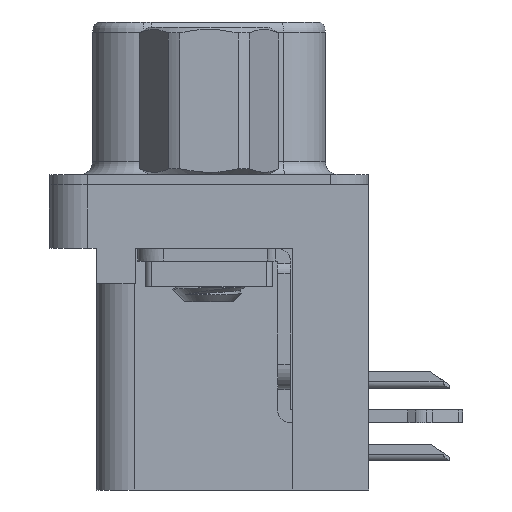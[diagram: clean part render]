
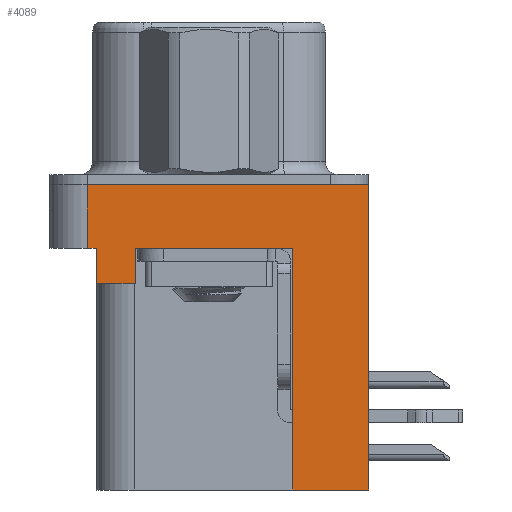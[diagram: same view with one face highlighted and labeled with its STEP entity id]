
A CAD part, left-side view. The second image highlights one B-rep face of the part: STEP entity #4089.
In plain terms, the highlighted planar face has unit normal (-1, 0, 0).
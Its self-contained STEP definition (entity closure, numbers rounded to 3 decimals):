
#299 = VECTOR ( 'NONE', #5499, 1000. ) ;
#328 = CARTESIAN_POINT ( 'NONE',  ( -2.935, -3.295, -12. ) ) ;
#560 = LINE ( 'NONE', #13703, #13429 ) ;
#997 = EDGE_CURVE ( 'NONE', #20167, #11208, #11952, .T. ) ;
#1249 = EDGE_CURVE ( 'NONE', #15625, #7028, #13150, .T. ) ;
#1356 = CARTESIAN_POINT ( 'NONE',  ( -2.935, 2.895, -2.5 ) ) ;
#1604 = CARTESIAN_POINT ( 'NONE',  ( -2.935, 2.895, -3.9 ) ) ;
#2336 = FACE_OUTER_BOUND ( 'NONE', #5915, .T. ) ;
#2530 = LINE ( 'NONE', #23417, #11788 ) ;
#2754 = ORIENTED_EDGE ( 'NONE', *, *, #14510, .F. ) ;
#2877 = VERTEX_POINT ( 'NONE', #21437 ) ;
#2952 = CARTESIAN_POINT ( 'NONE',  ( -2.935, -6.275, -2.5 ) ) ;
#3933 = ORIENTED_EDGE ( 'NONE', *, *, #22771, .F. ) ;
#4046 = EDGE_CURVE ( 'NONE', #7547, #11208, #22954, .T. ) ;
#4089 = ADVANCED_FACE ( 'NONE', ( #2336 ), #18401, .T. ) ;
#4191 = CARTESIAN_POINT ( 'NONE',  ( -2.935, -3.295, -2.5 ) ) ;
#4959 = CARTESIAN_POINT ( 'NONE',  ( -2.935, -6.275, -2.5 ) ) ;
#5136 = ORIENTED_EDGE ( 'NONE', *, *, #6308, .F. ) ;
#5379 = CARTESIAN_POINT ( 'NONE',  ( -2.935, 4.775, -2.5 ) ) ;
#5499 = DIRECTION ( 'NONE',  ( 0., 0., 1. ) ) ;
#5915 = EDGE_LOOP ( 'NONE', ( #3933, #5136, #23960, #6730, #2754, #13331, #23735, #17203, #6239, #22960 ) ) ;
#6004 = VERTEX_POINT ( 'NONE', #24434 ) ;
#6239 = ORIENTED_EDGE ( 'NONE', *, *, #7039, .F. ) ;
#6308 = EDGE_CURVE ( 'NONE', #20167, #7839, #18441, .T. ) ;
#6730 = ORIENTED_EDGE ( 'NONE', *, *, #4046, .F. ) ;
#6802 = CARTESIAN_POINT ( 'NONE',  ( -2.935, 4.425, -3.9 ) ) ;
#6884 = LINE ( 'NONE', #10600, #10438 ) ;
#7028 = VERTEX_POINT ( 'NONE', #4191 ) ;
#7034 = DIRECTION ( 'NONE',  ( -1., 0., 0. ) ) ;
#7039 = EDGE_CURVE ( 'NONE', #6004, #15625, #18699, .T. ) ;
#7547 = VERTEX_POINT ( 'NONE', #24356 ) ;
#7561 = LINE ( 'NONE', #18703, #10229 ) ;
#7839 = VERTEX_POINT ( 'NONE', #19649 ) ;
#8260 = VECTOR ( 'NONE', #24479, 1000. ) ;
#8465 = DIRECTION ( 'NONE',  ( 0., -1., 0. ) ) ;
#8544 = CARTESIAN_POINT ( 'NONE',  ( -2.935, 4.425, -3.9 ) ) ;
#8864 = DIRECTION ( 'NONE',  ( 0., 0., 1. ) ) ;
#9310 = EDGE_CURVE ( 'NONE', #11358, #7028, #7561, .T. ) ;
#9725 = VECTOR ( 'NONE', #17567, 1000. ) ;
#10229 = VECTOR ( 'NONE', #14680, 1000. ) ;
#10438 = VECTOR ( 'NONE', #23989, 1000. ) ;
#10600 = CARTESIAN_POINT ( 'NONE',  ( -2.935, 2.895, -3.9 ) ) ;
#11208 = VERTEX_POINT ( 'NONE', #15822 ) ;
#11358 = VERTEX_POINT ( 'NONE', #1356 ) ;
#11457 = EDGE_CURVE ( 'NONE', #6004, #2877, #560, .T. ) ;
#11788 = VECTOR ( 'NONE', #14001, 1000. ) ;
#11804 = EDGE_CURVE ( 'NONE', #11932, #11358, #6884, .T. ) ;
#11932 = VERTEX_POINT ( 'NONE', #1604 ) ;
#11952 = LINE ( 'NONE', #2952, #21549 ) ;
#11995 = LINE ( 'NONE', #8544, #21276 ) ;
#12116 = DIRECTION ( 'NONE',  ( 0., 0., 1. ) ) ;
#12714 = DIRECTION ( 'NONE',  ( 0., 0., 1. ) ) ;
#12791 = CARTESIAN_POINT ( 'NONE',  ( -2.935, 4.775, -2.5 ) ) ;
#13150 = LINE ( 'NONE', #16955, #299 ) ;
#13331 = ORIENTED_EDGE ( 'NONE', *, *, #11804, .T. ) ;
#13429 = VECTOR ( 'NONE', #12116, 1000. ) ;
#13703 = CARTESIAN_POINT ( 'NONE',  ( -2.935, -6.275, -2.5 ) ) ;
#14001 = DIRECTION ( 'NONE',  ( 0., -1., 0. ) ) ;
#14128 = DIRECTION ( 'NONE',  ( 0., 1., 0. ) ) ;
#14510 = EDGE_CURVE ( 'NONE', #11932, #7547, #11995, .T. ) ;
#14680 = DIRECTION ( 'NONE',  ( 0., -1., 0. ) ) ;
#15625 = VERTEX_POINT ( 'NONE', #21773 ) ;
#15822 = CARTESIAN_POINT ( 'NONE',  ( -2.935, 4.425, -2.5 ) ) ;
#16955 = CARTESIAN_POINT ( 'NONE',  ( -2.935, -3.295, -12. ) ) ;
#17203 = ORIENTED_EDGE ( 'NONE', *, *, #1249, .F. ) ;
#17567 = DIRECTION ( 'NONE',  ( 0., 1., 0. ) ) ;
#18401 = PLANE ( 'NONE',  #24238 ) ;
#18441 = LINE ( 'NONE', #5379, #8260 ) ;
#18699 = LINE ( 'NONE', #328, #9725 ) ;
#18703 = CARTESIAN_POINT ( 'NONE',  ( -2.935, -6.275, -2.5 ) ) ;
#19649 = CARTESIAN_POINT ( 'NONE',  ( -2.935, 4.775, 0. ) ) ;
#20167 = VERTEX_POINT ( 'NONE', #12791 ) ;
#21276 = VECTOR ( 'NONE', #14128, 1000. ) ;
#21437 = CARTESIAN_POINT ( 'NONE',  ( -2.935, -6.275, 0. ) ) ;
#21549 = VECTOR ( 'NONE', #8465, 1000. ) ;
#21773 = CARTESIAN_POINT ( 'NONE',  ( -2.935, -3.295, -12. ) ) ;
#22771 = EDGE_CURVE ( 'NONE', #7839, #2877, #2530, .T. ) ;
#22954 = LINE ( 'NONE', #6802, #23824 ) ;
#22960 = ORIENTED_EDGE ( 'NONE', *, *, #11457, .T. ) ;
#23417 = CARTESIAN_POINT ( 'NONE',  ( -2.935, -6.275, 0. ) ) ;
#23735 = ORIENTED_EDGE ( 'NONE', *, *, #9310, .T. ) ;
#23824 = VECTOR ( 'NONE', #8864, 1000. ) ;
#23960 = ORIENTED_EDGE ( 'NONE', *, *, #997, .T. ) ;
#23989 = DIRECTION ( 'NONE',  ( 0., 0., 1. ) ) ;
#24238 = AXIS2_PLACEMENT_3D ( 'NONE', #4959, #7034, #12714 ) ;
#24356 = CARTESIAN_POINT ( 'NONE',  ( -2.935, 4.425, -3.9 ) ) ;
#24434 = CARTESIAN_POINT ( 'NONE',  ( -2.935, -6.275, -12. ) ) ;
#24479 = DIRECTION ( 'NONE',  ( 0., 0., 1. ) ) ;
